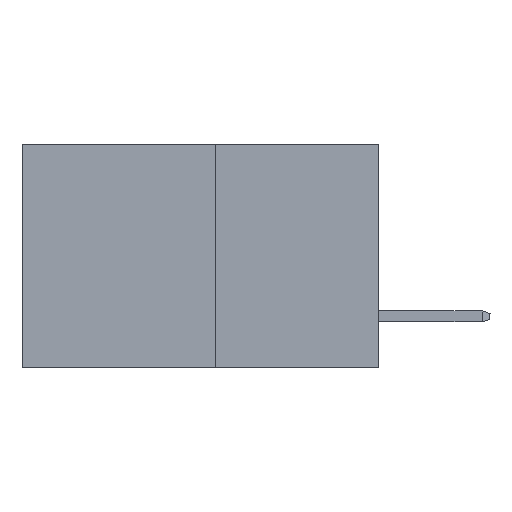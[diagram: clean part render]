
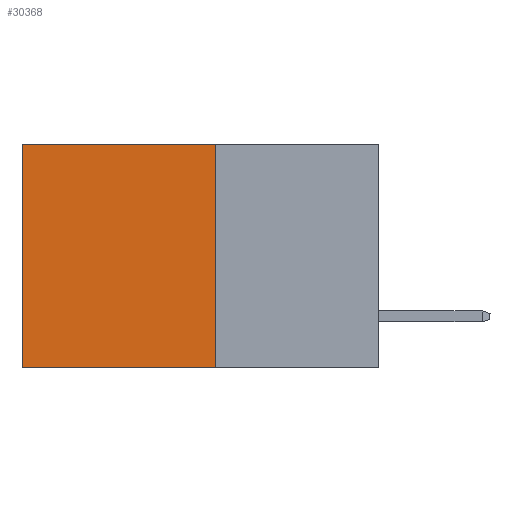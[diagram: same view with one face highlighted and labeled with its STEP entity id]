
A CAD part, left-side view. The second image highlights one B-rep face of the part: STEP entity #30368.
In plain terms, the highlighted planar face has unit normal (-1, 0, 0).
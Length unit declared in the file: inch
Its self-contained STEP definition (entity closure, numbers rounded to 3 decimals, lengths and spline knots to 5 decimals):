
#2343 = VERTEX_POINT ( 'NONE', #25149 ) ;
#3771 = EDGE_CURVE ( 'NONE', #2343, #13017, #6150, .T. ) ;
#3907 = DIRECTION ( 'NONE',  ( 1., 0., 0. ) ) ;
#4633 = CARTESIAN_POINT ( 'NONE',  ( 0.277, 0.59, 0. ) ) ;
#4728 = EDGE_LOOP ( 'NONE', ( #11733, #27765, #8665, #18861 ) ) ;
#6150 = LINE ( 'NONE', #25201, #22776 ) ;
#7348 = VERTEX_POINT ( 'NONE', #25778 ) ;
#7611 = AXIS2_PLACEMENT_3D ( 'NONE', #18018, #3907, #20379 ) ;
#7643 = DIRECTION ( 'NONE',  ( 0., 0., -1. ) ) ;
#7704 = CARTESIAN_POINT ( 'NONE',  ( 0.277, 0.27, -0.37 ) ) ;
#8074 = LINE ( 'NONE', #12326, #19864 ) ;
#8665 = ORIENTED_EDGE ( 'NONE', *, *, #11103, .F. ) ;
#11103 = EDGE_CURVE ( 'NONE', #2343, #7348, #26250, .T. ) ;
#11733 = ORIENTED_EDGE ( 'NONE', *, *, #16522, .T. ) ;
#12326 = CARTESIAN_POINT ( 'NONE',  ( 0.277, 0.59, -0.37 ) ) ;
#13017 = VERTEX_POINT ( 'NONE', #4633 ) ;
#13740 = FACE_OUTER_BOUND ( 'NONE', #4728, .T. ) ;
#14628 = DIRECTION ( 'NONE',  ( 0., 1., 0. ) ) ;
#16318 = LINE ( 'NONE', #21683, #29701 ) ;
#16522 = EDGE_CURVE ( 'NONE', #13017, #17332, #8074, .T. ) ;
#17332 = VERTEX_POINT ( 'NONE', #26913 ) ;
#18018 = CARTESIAN_POINT ( 'NONE',  ( 0.277, 0.27, -0.37 ) ) ;
#18861 = ORIENTED_EDGE ( 'NONE', *, *, #3771, .T. ) ;
#19849 = VECTOR ( 'NONE', #7643, 39.37008 ) ;
#19864 = VECTOR ( 'NONE', #21819, 39.37008 ) ;
#20379 = DIRECTION ( 'NONE',  ( 0., 0., -1. ) ) ;
#21683 = CARTESIAN_POINT ( 'NONE',  ( 0.277, 0.27, -0.37 ) ) ;
#21819 = DIRECTION ( 'NONE',  ( 0., 0., -1. ) ) ;
#22776 = VECTOR ( 'NONE', #22867, 39.37008 ) ;
#22867 = DIRECTION ( 'NONE',  ( 0., 1., 0. ) ) ;
#25147 = PLANE ( 'NONE',  #7611 ) ;
#25149 = CARTESIAN_POINT ( 'NONE',  ( 0.277, 0.27, 0. ) ) ;
#25201 = CARTESIAN_POINT ( 'NONE',  ( 0.277, 0.27, 0. ) ) ;
#25778 = CARTESIAN_POINT ( 'NONE',  ( 0.277, 0.27, -0.37 ) ) ;
#26250 = LINE ( 'NONE', #7704, #19849 ) ;
#26913 = CARTESIAN_POINT ( 'NONE',  ( 0.277, 0.59, -0.37 ) ) ;
#27765 = ORIENTED_EDGE ( 'NONE', *, *, #30104, .F. ) ;
#29701 = VECTOR ( 'NONE', #14628, 39.37008 ) ;
#30104 = EDGE_CURVE ( 'NONE', #7348, #17332, #16318, .T. ) ;
#30368 = ADVANCED_FACE ( 'NONE', ( #13740 ), #25147, .F. ) ;
